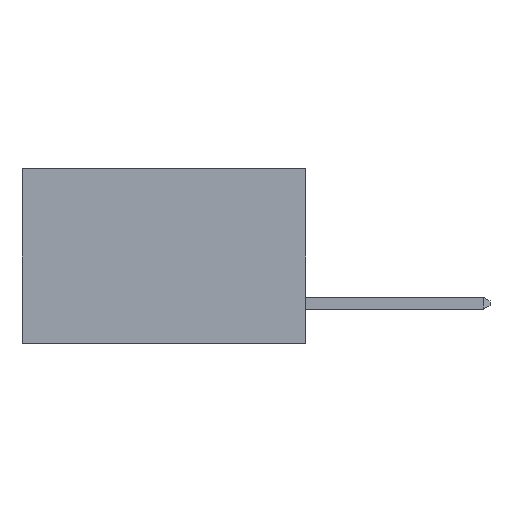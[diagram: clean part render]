
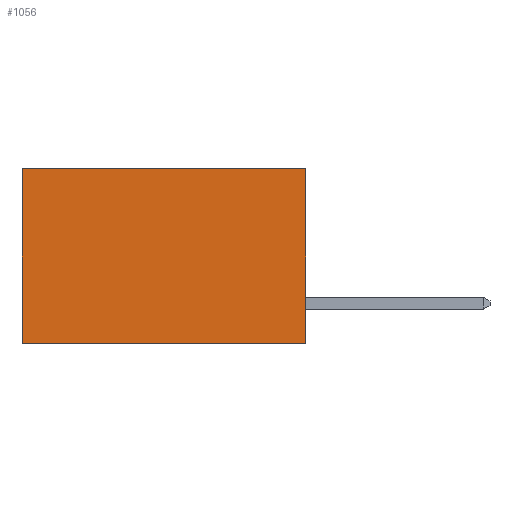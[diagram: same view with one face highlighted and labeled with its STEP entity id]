
A CAD part, left-side view. The second image highlights one B-rep face of the part: STEP entity #1056.
In plain terms, the highlighted planar face has unit normal (-1, 0, 0).
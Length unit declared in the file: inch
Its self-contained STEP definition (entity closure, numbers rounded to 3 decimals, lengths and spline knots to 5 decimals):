
#192 = EDGE_CURVE ( 'NONE', #3958, #2337, #7606, .T. ) ;
#208 = VECTOR ( 'NONE', #1128, 39.37008 ) ;
#487 = CARTESIAN_POINT ( 'NONE',  ( 0.2615, 0.6, 0. ) ) ;
#587 = ORIENTED_EDGE ( 'NONE', *, *, #5333, .T. ) ;
#734 = ORIENTED_EDGE ( 'NONE', *, *, #5742, .F. ) ;
#820 = ORIENTED_EDGE ( 'NONE', *, *, #192, .F. ) ;
#864 = DIRECTION ( 'NONE',  ( 0., 0., -1. ) ) ;
#878 = ORIENTED_EDGE ( 'NONE', *, *, #5322, .T. ) ;
#1056 = ADVANCED_FACE ( 'NONE', ( #8012 ), #3776, .F. ) ;
#1128 = DIRECTION ( 'NONE',  ( 0., 1., 0. ) ) ;
#1229 = CARTESIAN_POINT ( 'NONE',  ( 0.2615, 0., -0.37 ) ) ;
#1387 = VERTEX_POINT ( 'NONE', #487 ) ;
#1652 = LINE ( 'NONE', #3010, #8866 ) ;
#1839 = VECTOR ( 'NONE', #864, 39.37008 ) ;
#2337 = VERTEX_POINT ( 'NONE', #7470 ) ;
#2385 = LINE ( 'NONE', #6234, #208 ) ;
#2409 = CARTESIAN_POINT ( 'NONE',  ( 0.2615, 0., -0.37 ) ) ;
#2639 = EDGE_LOOP ( 'NONE', ( #587, #734, #820, #878 ) ) ;
#2651 = DIRECTION ( 'NONE',  ( 1., 0., 0. ) ) ;
#2934 = CARTESIAN_POINT ( 'NONE',  ( 0.2615, 0.6, -0.37 ) ) ;
#3010 = CARTESIAN_POINT ( 'NONE',  ( 0.2615, 0.6, -0.37 ) ) ;
#3776 = PLANE ( 'NONE',  #6809 ) ;
#3958 = VERTEX_POINT ( 'NONE', #4101 ) ;
#4101 = CARTESIAN_POINT ( 'NONE',  ( 0.2615, 0., 0. ) ) ;
#5084 = DIRECTION ( 'NONE',  ( 0., 0., -1. ) ) ;
#5322 = EDGE_CURVE ( 'NONE', #3958, #1387, #2385, .T. ) ;
#5333 = EDGE_CURVE ( 'NONE', #1387, #5488, #1652, .T. ) ;
#5488 = VERTEX_POINT ( 'NONE', #2934 ) ;
#5729 = VECTOR ( 'NONE', #8369, 39.37008 ) ;
#5742 = EDGE_CURVE ( 'NONE', #2337, #5488, #7852, .T. ) ;
#6234 = CARTESIAN_POINT ( 'NONE',  ( 0.2615, 0., 0. ) ) ;
#6809 = AXIS2_PLACEMENT_3D ( 'NONE', #2409, #2651, #5084 ) ;
#7470 = CARTESIAN_POINT ( 'NONE',  ( 0.2615, 0., -0.37 ) ) ;
#7606 = LINE ( 'NONE', #1229, #1839 ) ;
#7852 = LINE ( 'NONE', #9185, #5729 ) ;
#8012 = FACE_OUTER_BOUND ( 'NONE', #2639, .T. ) ;
#8369 = DIRECTION ( 'NONE',  ( 0., 1., 0. ) ) ;
#8866 = VECTOR ( 'NONE', #9413, 39.37008 ) ;
#9185 = CARTESIAN_POINT ( 'NONE',  ( 0.2615, 0., -0.37 ) ) ;
#9413 = DIRECTION ( 'NONE',  ( 0., 0., -1. ) ) ;
